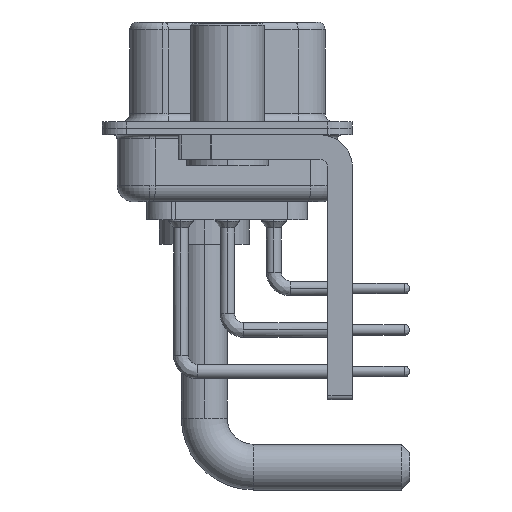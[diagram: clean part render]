
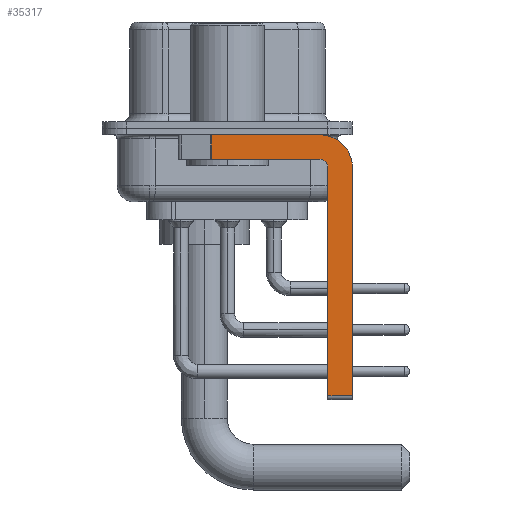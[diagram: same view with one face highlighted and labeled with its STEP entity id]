
A CAD part, left-side view. The second image highlights one B-rep face of the part: STEP entity #35317.
In plain terms, the highlighted planar face has unit normal (-1, 0, 0).
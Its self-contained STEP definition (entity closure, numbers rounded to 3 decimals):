
#47 = DIRECTION ( 'NONE',  ( -1., 0., 0. ) ) ;
#408 = CARTESIAN_POINT ( 'NONE',  ( -2.9, -7.65, -16.35 ) ) ;
#455 = CARTESIAN_POINT ( 'NONE',  ( -2.9, -5.65, -1.9 ) ) ;
#1911 = EDGE_CURVE ( 'NONE', #32116, #23162, #15896, .T. ) ;
#2745 = CARTESIAN_POINT ( 'NONE',  ( -2.9, -6.15, -16.35 ) ) ;
#3292 = EDGE_CURVE ( 'NONE', #15861, #37829, #10967, .T. ) ;
#3770 = CARTESIAN_POINT ( 'NONE',  ( -2.9, -5.65, -16.35 ) ) ;
#4340 = DIRECTION ( 'NONE',  ( 0., 0., -1. ) ) ;
#4777 = EDGE_CURVE ( 'NONE', #32116, #6636, #22567, .T. ) ;
#4807 = DIRECTION ( 'NONE',  ( 0., 0., -1. ) ) ;
#4901 = CARTESIAN_POINT ( 'NONE',  ( -2.9, -7.65, -2.4 ) ) ;
#5302 = AXIS2_PLACEMENT_3D ( 'NONE', #30722, #47, #36175 ) ;
#5491 = CARTESIAN_POINT ( 'NONE',  ( -2.9, 0.978, -0.4 ) ) ;
#6636 = VERTEX_POINT ( 'NONE', #27632 ) ;
#7393 = VERTEX_POINT ( 'NONE', #5491 ) ;
#7847 = ORIENTED_EDGE ( 'NONE', *, *, #3292, .F. ) ;
#8037 = FACE_OUTER_BOUND ( 'NONE', #27999, .T. ) ;
#9482 = AXIS2_PLACEMENT_3D ( 'NONE', #20387, #39157, #30261 ) ;
#10254 = CARTESIAN_POINT ( 'NONE',  ( -2.9, 0.978, -1.9 ) ) ;
#10766 = DIRECTION ( 'NONE',  ( 0., 1., 0. ) ) ;
#10967 = LINE ( 'NONE', #13819, #22502 ) ;
#11608 = ORIENTED_EDGE ( 'NONE', *, *, #1911, .T. ) ;
#11632 = ORIENTED_EDGE ( 'NONE', *, *, #4777, .F. ) ;
#12850 = DIRECTION ( 'NONE',  ( 0., -1., 0. ) ) ;
#13495 = VERTEX_POINT ( 'NONE', #36238 ) ;
#13819 = CARTESIAN_POINT ( 'NONE',  ( -2.9, -5.65, -1.9 ) ) ;
#15861 = VERTEX_POINT ( 'NONE', #455 ) ;
#15896 = LINE ( 'NONE', #3770, #26734 ) ;
#17028 = VERTEX_POINT ( 'NONE', #35599 ) ;
#18825 = ORIENTED_EDGE ( 'NONE', *, *, #32935, .F. ) ;
#18938 = CARTESIAN_POINT ( 'NONE',  ( -2.9, 0.978, -1.9 ) ) ;
#19484 = CIRCLE ( 'NONE', #5302, 0.5 ) ;
#19938 = DIRECTION ( 'NONE',  ( 0., 0., 1. ) ) ;
#20070 = CARTESIAN_POINT ( 'NONE',  ( -2.9, -5.65, -2.4 ) ) ;
#20387 = CARTESIAN_POINT ( 'NONE',  ( -2.9, -5.65, -2.4 ) ) ;
#20648 = DIRECTION ( 'NONE',  ( 0., 0., -1. ) ) ;
#22376 = CARTESIAN_POINT ( 'NONE',  ( -2.9, -6.15, -16.6 ) ) ;
#22502 = VECTOR ( 'NONE', #10766, 1000. ) ;
#22567 = LINE ( 'NONE', #22376, #39340 ) ;
#22927 = ORIENTED_EDGE ( 'NONE', *, *, #27422, .F. ) ;
#23162 = VERTEX_POINT ( 'NONE', #408 ) ;
#24150 = AXIS2_PLACEMENT_3D ( 'NONE', #20070, #34811, #4340 ) ;
#26212 = LINE ( 'NONE', #10254, #35535 ) ;
#26734 = VECTOR ( 'NONE', #12850, 1000. ) ;
#26849 = PLANE ( 'NONE',  #9482 ) ;
#27320 = LINE ( 'NONE', #33385, #33672 ) ;
#27422 = EDGE_CURVE ( 'NONE', #6636, #15861, #19484, .T. ) ;
#27632 = CARTESIAN_POINT ( 'NONE',  ( -2.9, -6.15, -2.4 ) ) ;
#27999 = EDGE_LOOP ( 'NONE', ( #32013, #35637, #7847, #22927, #11632, #11608, #35314, #18825 ) ) ;
#28127 = EDGE_CURVE ( 'NONE', #7393, #37829, #26212, .T. ) ;
#28690 = CIRCLE ( 'NONE', #24150, 2. ) ;
#29128 = LINE ( 'NONE', #4901, #39785 ) ;
#30261 = DIRECTION ( 'NONE',  ( 0., 0., -1. ) ) ;
#30493 = EDGE_CURVE ( 'NONE', #7393, #17028, #27320, .T. ) ;
#30722 = CARTESIAN_POINT ( 'NONE',  ( -2.9, -5.65, -2.4 ) ) ;
#32013 = ORIENTED_EDGE ( 'NONE', *, *, #30493, .F. ) ;
#32116 = VERTEX_POINT ( 'NONE', #2745 ) ;
#32935 = EDGE_CURVE ( 'NONE', #17028, #13495, #28690, .T. ) ;
#33385 = CARTESIAN_POINT ( 'NONE',  ( -2.9, 3., -0.4 ) ) ;
#33672 = VECTOR ( 'NONE', #35796, 1000. ) ;
#34811 = DIRECTION ( 'NONE',  ( 1., 0., 0. ) ) ;
#35314 = ORIENTED_EDGE ( 'NONE', *, *, #36529, .F. ) ;
#35317 = ADVANCED_FACE ( 'NONE', ( #8037 ), #26849, .F. ) ;
#35535 = VECTOR ( 'NONE', #4807, 1000. ) ;
#35599 = CARTESIAN_POINT ( 'NONE',  ( -2.9, -5.65, -0.4 ) ) ;
#35637 = ORIENTED_EDGE ( 'NONE', *, *, #28127, .T. ) ;
#35796 = DIRECTION ( 'NONE',  ( 0., -1., 0. ) ) ;
#36175 = DIRECTION ( 'NONE',  ( 0., 0., 1. ) ) ;
#36238 = CARTESIAN_POINT ( 'NONE',  ( -2.9, -7.65, -2.4 ) ) ;
#36529 = EDGE_CURVE ( 'NONE', #13495, #23162, #29128, .T. ) ;
#37829 = VERTEX_POINT ( 'NONE', #18938 ) ;
#39157 = DIRECTION ( 'NONE',  ( 1., 0., 0. ) ) ;
#39340 = VECTOR ( 'NONE', #19938, 1000. ) ;
#39785 = VECTOR ( 'NONE', #20648, 1000. ) ;
